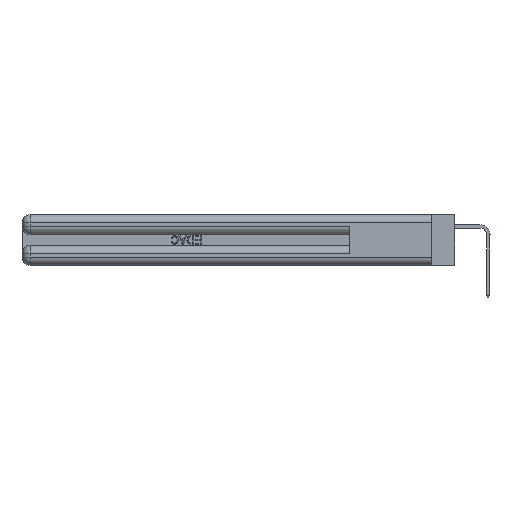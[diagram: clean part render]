
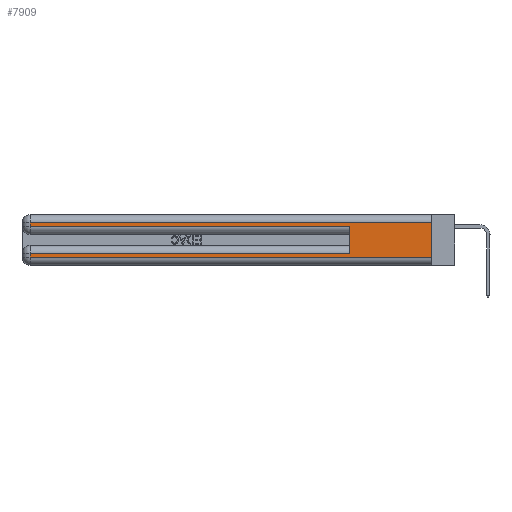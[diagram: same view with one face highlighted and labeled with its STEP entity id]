
A CAD part, left-side view. The second image highlights one B-rep face of the part: STEP entity #7909.
In plain terms, the highlighted planar face has unit normal (-1, 0, 0).
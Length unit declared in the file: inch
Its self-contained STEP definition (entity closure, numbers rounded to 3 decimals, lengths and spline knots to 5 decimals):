
#182 = CARTESIAN_POINT ( 'NONE',  ( 0., 2.94, 0.06 ) ) ;
#659 = VERTEX_POINT ( 'NONE', #40833 ) ;
#662 = LINE ( 'NONE', #35821, #8203 ) ;
#743 = LINE ( 'NONE', #24654, #25543 ) ;
#1339 = DIRECTION ( 'NONE',  ( 0., 0., -1. ) ) ;
#2840 = EDGE_CURVE ( 'NONE', #38368, #30869, #9253, .T. ) ;
#3240 = DIRECTION ( 'NONE',  ( 0., 1., 0. ) ) ;
#3502 = CARTESIAN_POINT ( 'NONE',  ( 0., 0., 0.37 ) ) ;
#3880 = DIRECTION ( 'NONE',  ( 0., 0., -1. ) ) ;
#4240 = ORIENTED_EDGE ( 'NONE', *, *, #12348, .T. ) ;
#4541 = ORIENTED_EDGE ( 'NONE', *, *, #11516, .T. ) ;
#5679 = VERTEX_POINT ( 'NONE', #32596 ) ;
#5898 = AXIS2_PLACEMENT_3D ( 'NONE', #3502, #13283, #35789 ) ;
#6010 = LINE ( 'NONE', #26548, #22292 ) ;
#6767 = ORIENTED_EDGE ( 'NONE', *, *, #40271, .T. ) ;
#7780 = FACE_OUTER_BOUND ( 'NONE', #9960, .T. ) ;
#7909 = ADVANCED_FACE ( 'NONE', ( #7780 ), #9990, .F. ) ;
#8203 = VECTOR ( 'NONE', #19850, 39.37008 ) ;
#9253 = LINE ( 'NONE', #36394, #41394 ) ;
#9960 = EDGE_LOOP ( 'NONE', ( #34029, #11321, #4240, #12396, #39974, #6767, #19252, #4541 ) ) ;
#9990 = PLANE ( 'NONE',  #5898 ) ;
#10614 = VERTEX_POINT ( 'NONE', #17060 ) ;
#10734 = CARTESIAN_POINT ( 'NONE',  ( 0., 0.6, 0.085 ) ) ;
#11321 = ORIENTED_EDGE ( 'NONE', *, *, #41056, .T. ) ;
#11391 = LINE ( 'NONE', #30192, #20038 ) ;
#11516 = EDGE_CURVE ( 'NONE', #36431, #10614, #743, .T. ) ;
#12348 = EDGE_CURVE ( 'NONE', #14343, #12932, #662, .T. ) ;
#12396 = ORIENTED_EDGE ( 'NONE', *, *, #23210, .T. ) ;
#12932 = VERTEX_POINT ( 'NONE', #16797 ) ;
#13283 = DIRECTION ( 'NONE',  ( 1., 0., 0. ) ) ;
#13687 = EDGE_CURVE ( 'NONE', #659, #36431, #25349, .T. ) ;
#14343 = VERTEX_POINT ( 'NONE', #23942 ) ;
#14867 = LINE ( 'NONE', #28197, #31025 ) ;
#16797 = CARTESIAN_POINT ( 'NONE',  ( 0., 2.94, 0.285 ) ) ;
#17060 = CARTESIAN_POINT ( 'NONE',  ( 0., 0., 0.06 ) ) ;
#17145 = DIRECTION ( 'NONE',  ( 0., 0., 1. ) ) ;
#18117 = DIRECTION ( 'NONE',  ( 0., -1., 0. ) ) ;
#18525 = CARTESIAN_POINT ( 'NONE',  ( 0., 0.6, 0.285 ) ) ;
#19252 = ORIENTED_EDGE ( 'NONE', *, *, #13687, .T. ) ;
#19850 = DIRECTION ( 'NONE',  ( 0., 0., -1. ) ) ;
#20038 = VECTOR ( 'NONE', #33573, 39.37008 ) ;
#22292 = VECTOR ( 'NONE', #3880, 39.37008 ) ;
#23210 = EDGE_CURVE ( 'NONE', #12932, #30869, #14867, .T. ) ;
#23942 = CARTESIAN_POINT ( 'NONE',  ( 0., 2.94, 0.31 ) ) ;
#24654 = CARTESIAN_POINT ( 'NONE',  ( 0., 0., 0.06 ) ) ;
#25349 = LINE ( 'NONE', #27078, #31891 ) ;
#25543 = VECTOR ( 'NONE', #18117, 39.37008 ) ;
#25904 = CARTESIAN_POINT ( 'NONE',  ( 0., 0., 0.085 ) ) ;
#26548 = CARTESIAN_POINT ( 'NONE',  ( 0., 0., 0.37 ) ) ;
#27078 = CARTESIAN_POINT ( 'NONE',  ( 0., 2.94, 0.37 ) ) ;
#28197 = CARTESIAN_POINT ( 'NONE',  ( 0., 0., 0.285 ) ) ;
#30192 = CARTESIAN_POINT ( 'NONE',  ( 0., 0., 0.31 ) ) ;
#30869 = VERTEX_POINT ( 'NONE', #18525 ) ;
#31025 = VECTOR ( 'NONE', #40827, 39.37008 ) ;
#31891 = VECTOR ( 'NONE', #1339, 39.37008 ) ;
#32596 = CARTESIAN_POINT ( 'NONE',  ( 0., 0., 0.31 ) ) ;
#33573 = DIRECTION ( 'NONE',  ( 0., 1., 0. ) ) ;
#34029 = ORIENTED_EDGE ( 'NONE', *, *, #38939, .F. ) ;
#35789 = DIRECTION ( 'NONE',  ( 0., 0., -1. ) ) ;
#35821 = CARTESIAN_POINT ( 'NONE',  ( 0., 2.94, 0.37 ) ) ;
#36394 = CARTESIAN_POINT ( 'NONE',  ( 0., 0.6, 0.145 ) ) ;
#36431 = VERTEX_POINT ( 'NONE', #182 ) ;
#38368 = VERTEX_POINT ( 'NONE', #10734 ) ;
#38939 = EDGE_CURVE ( 'NONE', #5679, #10614, #6010, .T. ) ;
#39974 = ORIENTED_EDGE ( 'NONE', *, *, #2840, .F. ) ;
#40271 = EDGE_CURVE ( 'NONE', #38368, #659, #41557, .T. ) ;
#40558 = VECTOR ( 'NONE', #3240, 39.37008 ) ;
#40827 = DIRECTION ( 'NONE',  ( 0., -1., 0. ) ) ;
#40833 = CARTESIAN_POINT ( 'NONE',  ( 0., 2.94, 0.085 ) ) ;
#41056 = EDGE_CURVE ( 'NONE', #5679, #14343, #11391, .T. ) ;
#41394 = VECTOR ( 'NONE', #17145, 39.37008 ) ;
#41557 = LINE ( 'NONE', #25904, #40558 ) ;
